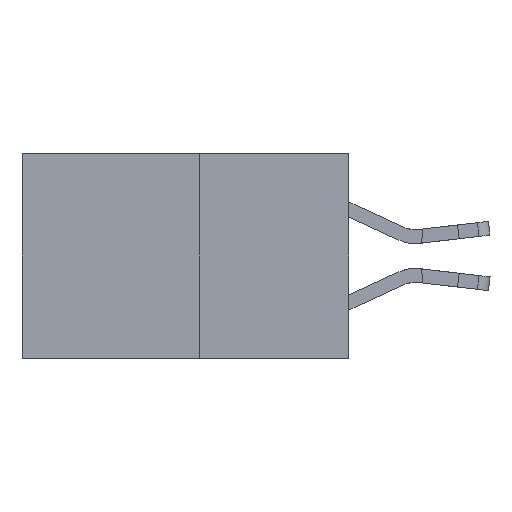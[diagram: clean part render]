
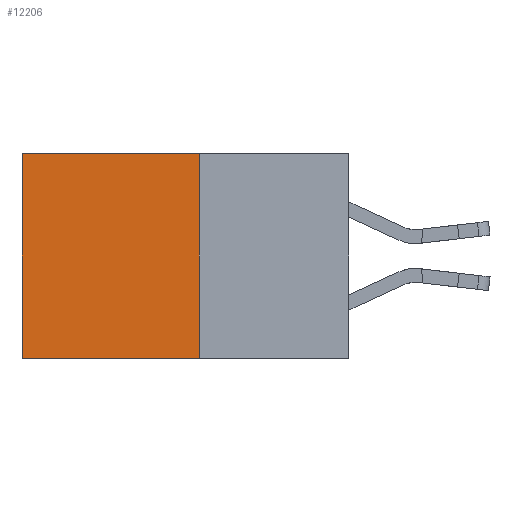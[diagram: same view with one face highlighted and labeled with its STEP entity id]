
A CAD part, left-side view. The second image highlights one B-rep face of the part: STEP entity #12206.
In plain terms, the highlighted planar face has unit normal (-1, 0, 0).
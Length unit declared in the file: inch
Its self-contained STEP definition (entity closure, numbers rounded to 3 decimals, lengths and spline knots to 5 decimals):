
#414 = DIRECTION ( 'NONE',  ( 0., 0., -1. ) ) ;
#807 = DIRECTION ( 'NONE',  ( 0., 1., 0. ) ) ;
#1717 = CARTESIAN_POINT ( 'NONE',  ( 0.277, 0.27, -0.37 ) ) ;
#2487 = LINE ( 'NONE', #1717, #9917 ) ;
#2906 = FACE_OUTER_BOUND ( 'NONE', #17369, .T. ) ;
#4274 = CARTESIAN_POINT ( 'NONE',  ( 0.277, 0.59, -0.37 ) ) ;
#4603 = EDGE_CURVE ( 'NONE', #13715, #15171, #12949, .T. ) ;
#5124 = ORIENTED_EDGE ( 'NONE', *, *, #4603, .T. ) ;
#5446 = VECTOR ( 'NONE', #807, 39.37008 ) ;
#5494 = CARTESIAN_POINT ( 'NONE',  ( 0.277, 0.27, -0.37 ) ) ;
#5830 = CARTESIAN_POINT ( 'NONE',  ( 0.277, 0.27, 0. ) ) ;
#6302 = DIRECTION ( 'NONE',  ( 0., 1., 0. ) ) ;
#6559 = LINE ( 'NONE', #5830, #17842 ) ;
#6652 = CARTESIAN_POINT ( 'NONE',  ( 0.277, 0.27, -0.37 ) ) ;
#7130 = CARTESIAN_POINT ( 'NONE',  ( 0.277, 0.27, 0. ) ) ;
#7397 = EDGE_CURVE ( 'NONE', #14275, #13715, #6559, .T. ) ;
#7717 = ORIENTED_EDGE ( 'NONE', *, *, #7397, .T. ) ;
#8504 = DIRECTION ( 'NONE',  ( 1., 0., 0. ) ) ;
#9421 = LINE ( 'NONE', #6652, #5446 ) ;
#9487 = VECTOR ( 'NONE', #414, 39.37008 ) ;
#9611 = VERTEX_POINT ( 'NONE', #10778 ) ;
#9917 = VECTOR ( 'NONE', #12078, 39.37008 ) ;
#10640 = CARTESIAN_POINT ( 'NONE',  ( 0.277, 0.59, -0.37 ) ) ;
#10778 = CARTESIAN_POINT ( 'NONE',  ( 0.277, 0.27, -0.37 ) ) ;
#11417 = PLANE ( 'NONE',  #14692 ) ;
#11775 = EDGE_CURVE ( 'NONE', #14275, #9611, #2487, .T. ) ;
#12078 = DIRECTION ( 'NONE',  ( 0., 0., -1. ) ) ;
#12206 = ADVANCED_FACE ( 'NONE', ( #2906 ), #11417, .F. ) ;
#12756 = EDGE_CURVE ( 'NONE', #9611, #15171, #9421, .T. ) ;
#12949 = LINE ( 'NONE', #10640, #9487 ) ;
#13715 = VERTEX_POINT ( 'NONE', #16259 ) ;
#14275 = VERTEX_POINT ( 'NONE', #7130 ) ;
#14692 = AXIS2_PLACEMENT_3D ( 'NONE', #5494, #8504, #18740 ) ;
#15171 = VERTEX_POINT ( 'NONE', #4274 ) ;
#16259 = CARTESIAN_POINT ( 'NONE',  ( 0.277, 0.59, 0. ) ) ;
#17369 = EDGE_LOOP ( 'NONE', ( #5124, #18249, #18033, #7717 ) ) ;
#17842 = VECTOR ( 'NONE', #6302, 39.37008 ) ;
#18033 = ORIENTED_EDGE ( 'NONE', *, *, #11775, .F. ) ;
#18249 = ORIENTED_EDGE ( 'NONE', *, *, #12756, .F. ) ;
#18740 = DIRECTION ( 'NONE',  ( 0., 0., -1. ) ) ;
